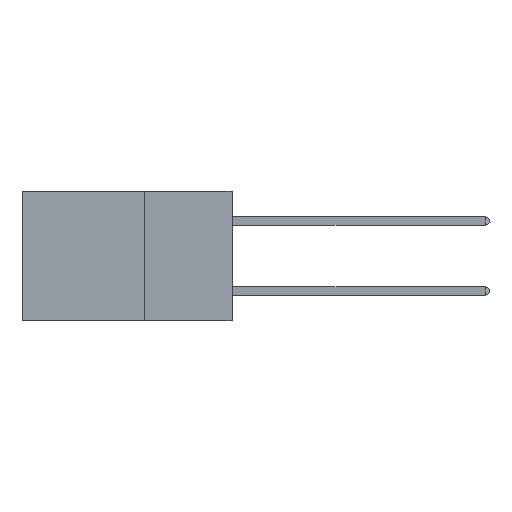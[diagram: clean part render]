
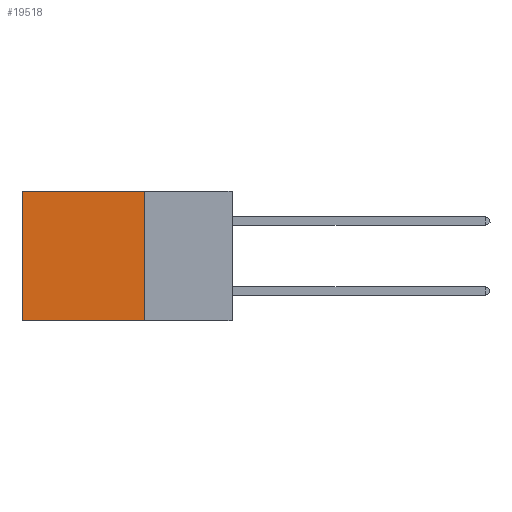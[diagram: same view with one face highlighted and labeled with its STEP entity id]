
A CAD part, left-side view. The second image highlights one B-rep face of the part: STEP entity #19518.
In plain terms, the highlighted planar face has unit normal (-1, 0, 0).
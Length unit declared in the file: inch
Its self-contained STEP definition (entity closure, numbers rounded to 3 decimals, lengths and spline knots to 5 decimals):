
#366 = VECTOR ( 'NONE', #22367, 39.37008 ) ;
#1957 = EDGE_CURVE ( 'NONE', #19130, #8571, #15405, .T. ) ;
#2385 = CARTESIAN_POINT ( 'NONE',  ( 0.2875, 0.6, 0. ) ) ;
#2535 = CARTESIAN_POINT ( 'NONE',  ( 0.2875, 0.25, 0. ) ) ;
#3436 = AXIS2_PLACEMENT_3D ( 'NONE', #2535, #16693, #9780 ) ;
#3650 = CARTESIAN_POINT ( 'NONE',  ( 0.2875, 0.25, 0. ) ) ;
#4257 = PLANE ( 'NONE',  #3436 ) ;
#5011 = ORIENTED_EDGE ( 'NONE', *, *, #22863, .F. ) ;
#5296 = VERTEX_POINT ( 'NONE', #12185 ) ;
#6350 = EDGE_LOOP ( 'NONE', ( #14997, #5011, #15809, #7402 ) ) ;
#7402 = ORIENTED_EDGE ( 'NONE', *, *, #20526, .T. ) ;
#8571 = VERTEX_POINT ( 'NONE', #9323 ) ;
#8792 = CARTESIAN_POINT ( 'NONE',  ( 0.2875, 0.25, 0. ) ) ;
#9001 = VECTOR ( 'NONE', #16740, 39.37008 ) ;
#9323 = CARTESIAN_POINT ( 'NONE',  ( 0.2875, 0.25, -0.37 ) ) ;
#9780 = DIRECTION ( 'NONE',  ( 0., 0., -1. ) ) ;
#9986 = CARTESIAN_POINT ( 'NONE',  ( 0.2875, 0.6, 0. ) ) ;
#10549 = VERTEX_POINT ( 'NONE', #2385 ) ;
#12185 = CARTESIAN_POINT ( 'NONE',  ( 0.2875, 0.6, -0.37 ) ) ;
#12376 = LINE ( 'NONE', #9986, #366 ) ;
#13318 = FACE_OUTER_BOUND ( 'NONE', #6350, .T. ) ;
#13994 = VECTOR ( 'NONE', #20790, 39.37008 ) ;
#14293 = LINE ( 'NONE', #17175, #13994 ) ;
#14924 = VECTOR ( 'NONE', #17736, 39.37008 ) ;
#14997 = ORIENTED_EDGE ( 'NONE', *, *, #22201, .T. ) ;
#15405 = LINE ( 'NONE', #22134, #9001 ) ;
#15809 = ORIENTED_EDGE ( 'NONE', *, *, #1957, .F. ) ;
#16693 = DIRECTION ( 'NONE',  ( 1., 0., 0. ) ) ;
#16740 = DIRECTION ( 'NONE',  ( 0., 0., -1. ) ) ;
#17175 = CARTESIAN_POINT ( 'NONE',  ( 0.2875, 0.25, -0.37 ) ) ;
#17736 = DIRECTION ( 'NONE',  ( 0., 1., 0. ) ) ;
#19114 = LINE ( 'NONE', #8792, #14924 ) ;
#19130 = VERTEX_POINT ( 'NONE', #3650 ) ;
#19518 = ADVANCED_FACE ( 'NONE', ( #13318 ), #4257, .F. ) ;
#20526 = EDGE_CURVE ( 'NONE', #19130, #10549, #19114, .T. ) ;
#20790 = DIRECTION ( 'NONE',  ( 0., 1., 0. ) ) ;
#22134 = CARTESIAN_POINT ( 'NONE',  ( 0.2875, 0.25, 0. ) ) ;
#22201 = EDGE_CURVE ( 'NONE', #10549, #5296, #12376, .T. ) ;
#22367 = DIRECTION ( 'NONE',  ( 0., 0., -1. ) ) ;
#22863 = EDGE_CURVE ( 'NONE', #8571, #5296, #14293, .T. ) ;
